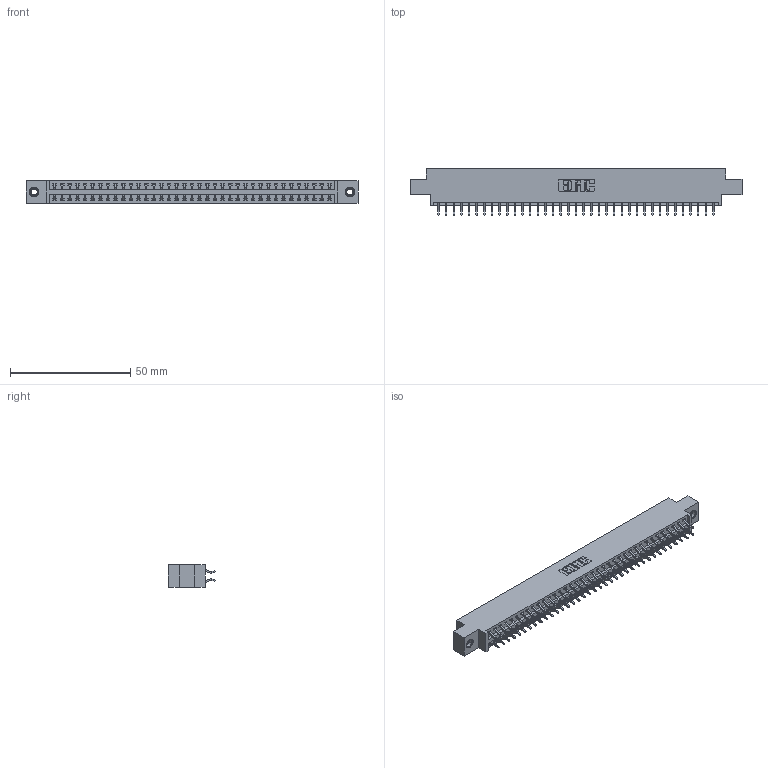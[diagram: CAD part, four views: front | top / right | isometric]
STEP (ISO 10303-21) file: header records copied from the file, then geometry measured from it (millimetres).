
FILE_DESCRIPTION (( 'STEP AP203' ), '1' );
FILE_NAME ('346-074-556-807.STEP', '2018-08-29T02:54:13', ( '' ), ( '' ), 'SwSTEP 2.0', 'SolidWorks 2016', '' );
FILE_SCHEMA (( 'CONFIG_CONTROL_DESIGN' ));
Length unit declared in the file: inch
Products named in the file (4): 346 Part_0.170 Offset - 0.156 Dia-TI; 345-292-001_556 Tail; 345-250-001_345-250-005-103; 346-074-556-807
Assembly tree (77 placements, depth 2):
  346-074-556-807
    346 Part_0.170 Offset - 0.156 Dia-TI
    345-292-001_556 Tail  x74
    345-250-001_345-250-005-103  x2
Bounding box: 138.05 x 19.57 x 9.4 mm (x, y, z)
Volume: 13251.6 mm3; surface area: 18281.3 mm2
Topology: 77 solids, 77 shells, 4478 faces, 13279 edges, 8746 vertices
Faces by surface type: plane 2998, cylinder 1464, cone 12, torus 4
Entity records: 26358 total; most frequent: CARTESIAN_POINT 4351, ORIENTED_EDGE 4266, DIRECTION 3899, EDGE_CURVE 2133, VECTOR 1825, LINE 1825, VERTEX_POINT 1416, AXIS2_PLACEMENT_3D 1037
